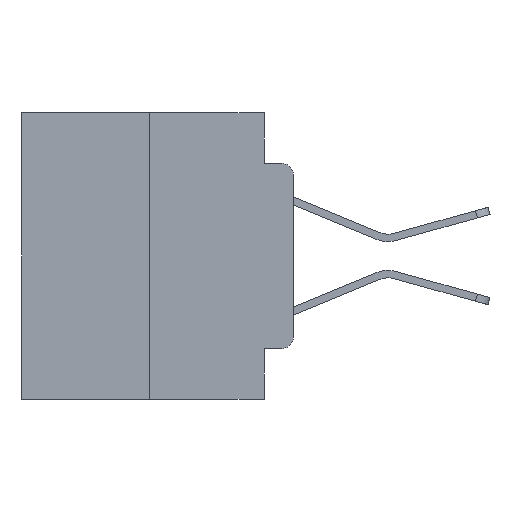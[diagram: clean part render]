
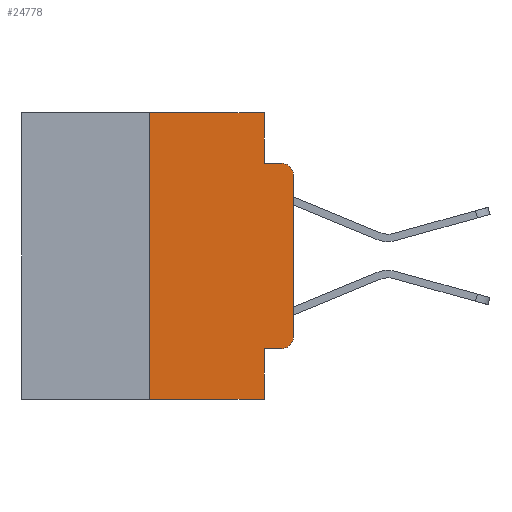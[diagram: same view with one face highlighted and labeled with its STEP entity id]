
A CAD part, left-side view. The second image highlights one B-rep face of the part: STEP entity #24778.
In plain terms, the highlighted planar face has unit normal (-1, 0, 0).
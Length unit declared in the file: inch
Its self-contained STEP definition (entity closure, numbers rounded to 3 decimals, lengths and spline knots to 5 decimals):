
#155 = CARTESIAN_POINT ( 'NONE',  ( 0., 0.051, -0.5 ) ) ;
#184 = DIRECTION ( 'NONE',  ( 0., 0., -1. ) ) ;
#710 = LINE ( 'NONE', #14555, #17492 ) ;
#858 = VERTEX_POINT ( 'NONE', #5382 ) ;
#958 = DIRECTION ( 'NONE',  ( 1., 0., 0. ) ) ;
#1181 = DIRECTION ( 'NONE',  ( 0., 0., 1. ) ) ;
#1932 = LINE ( 'NONE', #13659, #7159 ) ;
#2029 = VERTEX_POINT ( 'NONE', #18201 ) ;
#2477 = LINE ( 'NONE', #8559, #8399 ) ;
#3094 = DIRECTION ( 'NONE',  ( 0., 0., -1. ) ) ;
#3152 = CARTESIAN_POINT ( 'NONE',  ( 0., 0.051, 0. ) ) ;
#3442 = DIRECTION ( 'NONE',  ( 0., -1., 0. ) ) ;
#4308 = EDGE_CURVE ( 'NONE', #858, #22151, #22766, .T. ) ;
#4392 = CARTESIAN_POINT ( 'NONE',  ( 0., 0.051, 0. ) ) ;
#4795 = VECTOR ( 'NONE', #3094, 39.37008 ) ;
#5117 = VECTOR ( 'NONE', #3442, 39.37008 ) ;
#5209 = AXIS2_PLACEMENT_3D ( 'NONE', #11841, #26981, #14033 ) ;
#5272 = ORIENTED_EDGE ( 'NONE', *, *, #21753, .T. ) ;
#5382 = CARTESIAN_POINT ( 'NONE',  ( 0., 0.02, -0.4115 ) ) ;
#5576 = VERTEX_POINT ( 'NONE', #22389 ) ;
#5615 = ORIENTED_EDGE ( 'NONE', *, *, #17776, .T. ) ;
#5796 = EDGE_CURVE ( 'NONE', #27057, #858, #710, .T. ) ;
#6059 = AXIS2_PLACEMENT_3D ( 'NONE', #26369, #13407, #184 ) ;
#6610 = DIRECTION ( 'NONE',  ( 0., 0., -1. ) ) ;
#6924 = ORIENTED_EDGE ( 'NONE', *, *, #5796, .T. ) ;
#7104 = DIRECTION ( 'NONE',  ( 0., -1., 0. ) ) ;
#7119 = ORIENTED_EDGE ( 'NONE', *, *, #4308, .T. ) ;
#7159 = VECTOR ( 'NONE', #7104, 39.37008 ) ;
#7250 = EDGE_CURVE ( 'NONE', #27057, #22726, #24880, .T. ) ;
#7583 = PLANE ( 'NONE',  #10480 ) ;
#7684 = CARTESIAN_POINT ( 'NONE',  ( 0., 0.25, 0. ) ) ;
#7845 = CARTESIAN_POINT ( 'NONE',  ( 0., 0., 0. ) ) ;
#8126 = ORIENTED_EDGE ( 'NONE', *, *, #7250, .F. ) ;
#8263 = VERTEX_POINT ( 'NONE', #3152 ) ;
#8399 = VECTOR ( 'NONE', #13003, 39.37008 ) ;
#8559 = CARTESIAN_POINT ( 'NONE',  ( 0., 0.473, 0. ) ) ;
#10184 = EDGE_CURVE ( 'NONE', #24414, #10998, #24754, .T. ) ;
#10375 = CARTESIAN_POINT ( 'NONE',  ( 0., 0.25, -0.5 ) ) ;
#10480 = AXIS2_PLACEMENT_3D ( 'NONE', #20549, #958, #16282 ) ;
#10575 = FACE_OUTER_BOUND ( 'NONE', #11914, .T. ) ;
#10998 = VERTEX_POINT ( 'NONE', #7684 ) ;
#11144 = VERTEX_POINT ( 'NONE', #23289 ) ;
#11614 = EDGE_CURVE ( 'NONE', #8263, #2029, #27192, .T. ) ;
#11841 = CARTESIAN_POINT ( 'NONE',  ( 0., 0.02, -0.3915 ) ) ;
#11914 = EDGE_LOOP ( 'NONE', ( #5272, #15575, #14854, #14732, #13440, #12335, #5615, #8126, #6924, #7119 ) ) ;
#12335 = ORIENTED_EDGE ( 'NONE', *, *, #10184, .F. ) ;
#12465 = CIRCLE ( 'NONE', #6059, 0.02 ) ;
#13003 = DIRECTION ( 'NONE',  ( 0., -1., 0. ) ) ;
#13407 = DIRECTION ( 'NONE',  ( -1., 0., 0. ) ) ;
#13440 = ORIENTED_EDGE ( 'NONE', *, *, #27765, .F. ) ;
#13659 = CARTESIAN_POINT ( 'NONE',  ( 0., 0.473, -0.5 ) ) ;
#14033 = DIRECTION ( 'NONE',  ( 0., 0., -1. ) ) ;
#14555 = CARTESIAN_POINT ( 'NONE',  ( 0., 0.051, -0.4115 ) ) ;
#14732 = ORIENTED_EDGE ( 'NONE', *, *, #11614, .F. ) ;
#14747 = CARTESIAN_POINT ( 'NONE',  ( 0., 0.051, -0.4115 ) ) ;
#14854 = ORIENTED_EDGE ( 'NONE', *, *, #17406, .F. ) ;
#15575 = ORIENTED_EDGE ( 'NONE', *, *, #20306, .T. ) ;
#15577 = CARTESIAN_POINT ( 'NONE',  ( 0., 0., -0.3915 ) ) ;
#16282 = DIRECTION ( 'NONE',  ( 0., 0., -1. ) ) ;
#16479 = CARTESIAN_POINT ( 'NONE',  ( 0., 0.051, -0.0885 ) ) ;
#16525 = DIRECTION ( 'NONE',  ( 0., 0., 1. ) ) ;
#16665 = LINE ( 'NONE', #16479, #5117 ) ;
#17406 = EDGE_CURVE ( 'NONE', #2029, #5576, #16665, .T. ) ;
#17492 = VECTOR ( 'NONE', #18881, 39.37008 ) ;
#17776 = EDGE_CURVE ( 'NONE', #24414, #22726, #1932, .T. ) ;
#18124 = VECTOR ( 'NONE', #16525, 39.37008 ) ;
#18201 = CARTESIAN_POINT ( 'NONE',  ( 0., 0.051, -0.0885 ) ) ;
#18881 = DIRECTION ( 'NONE',  ( 0., -1., 0. ) ) ;
#19112 = VECTOR ( 'NONE', #6610, 39.37008 ) ;
#19649 = VECTOR ( 'NONE', #1181, 39.37008 ) ;
#20306 = EDGE_CURVE ( 'NONE', #11144, #5576, #12465, .T. ) ;
#20549 = CARTESIAN_POINT ( 'NONE',  ( 0., 0.473, 0. ) ) ;
#21753 = EDGE_CURVE ( 'NONE', #22151, #11144, #24595, .T. ) ;
#22151 = VERTEX_POINT ( 'NONE', #15577 ) ;
#22389 = CARTESIAN_POINT ( 'NONE',  ( 0., 0.02, -0.0885 ) ) ;
#22595 = CARTESIAN_POINT ( 'NONE',  ( 0., 0.051, 0. ) ) ;
#22726 = VERTEX_POINT ( 'NONE', #155 ) ;
#22766 = CIRCLE ( 'NONE', #5209, 0.02 ) ;
#23289 = CARTESIAN_POINT ( 'NONE',  ( 0., 0., -0.1085 ) ) ;
#24414 = VERTEX_POINT ( 'NONE', #10375 ) ;
#24595 = LINE ( 'NONE', #7845, #18124 ) ;
#24754 = LINE ( 'NONE', #27209, #19649 ) ;
#24778 = ADVANCED_FACE ( 'NONE', ( #10575 ), #7583, .F. ) ;
#24880 = LINE ( 'NONE', #4392, #19112 ) ;
#26369 = CARTESIAN_POINT ( 'NONE',  ( 0., 0.02, -0.1085 ) ) ;
#26981 = DIRECTION ( 'NONE',  ( -1., 0., 0. ) ) ;
#27057 = VERTEX_POINT ( 'NONE', #14747 ) ;
#27192 = LINE ( 'NONE', #22595, #4795 ) ;
#27209 = CARTESIAN_POINT ( 'NONE',  ( 0., 0.25, 0. ) ) ;
#27765 = EDGE_CURVE ( 'NONE', #10998, #8263, #2477, .T. ) ;
